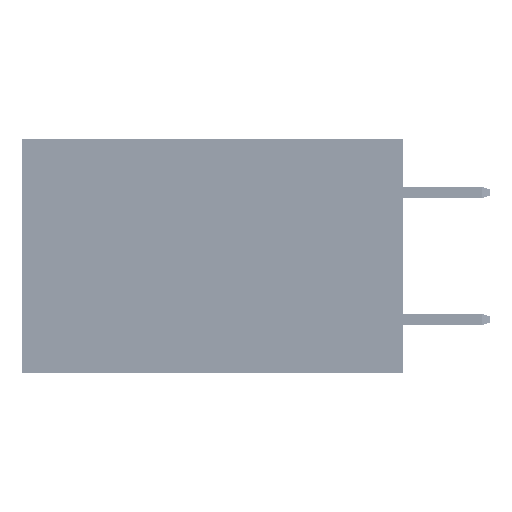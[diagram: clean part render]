
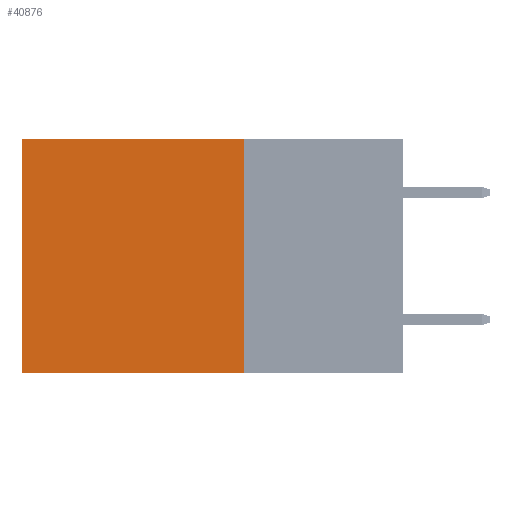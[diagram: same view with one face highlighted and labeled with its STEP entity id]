
A CAD part, left-side view. The second image highlights one B-rep face of the part: STEP entity #40876.
In plain terms, the highlighted planar face has unit normal (-1, 0, 0).
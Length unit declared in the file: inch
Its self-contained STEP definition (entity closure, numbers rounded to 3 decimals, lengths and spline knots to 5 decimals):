
#235 = VERTEX_POINT ( 'NONE', #27423 ) ;
#809 = EDGE_CURVE ( 'NONE', #15833, #235, #5172, .T. ) ;
#906 = CARTESIAN_POINT ( 'NONE',  ( 0.2875, 0.25, 0. ) ) ;
#944 = CARTESIAN_POINT ( 'NONE',  ( 0.2875, 0.25, 0. ) ) ;
#1489 = DIRECTION ( 'NONE',  ( 0., 0., -1. ) ) ;
#1515 = CARTESIAN_POINT ( 'NONE',  ( 0.2875, 0.25, -0.37 ) ) ;
#2453 = ORIENTED_EDGE ( 'NONE', *, *, #28197, .F. ) ;
#3823 = VERTEX_POINT ( 'NONE', #26135 ) ;
#4709 = LINE ( 'NONE', #1515, #15919 ) ;
#4826 = EDGE_LOOP ( 'NONE', ( #23606, #8934, #2453, #17939 ) ) ;
#5172 = LINE ( 'NONE', #35268, #29709 ) ;
#5693 = CARTESIAN_POINT ( 'NONE',  ( 0.2875, 0.25, 0. ) ) ;
#7968 = DIRECTION ( 'NONE',  ( 0., 0., -1. ) ) ;
#8451 = CARTESIAN_POINT ( 'NONE',  ( 0.2875, 0.25, 0. ) ) ;
#8521 = LINE ( 'NONE', #906, #23841 ) ;
#8934 = ORIENTED_EDGE ( 'NONE', *, *, #21193, .F. ) ;
#12122 = PLANE ( 'NONE',  #23232 ) ;
#14660 = VECTOR ( 'NONE', #19753, 39.37008 ) ;
#15833 = VERTEX_POINT ( 'NONE', #41503 ) ;
#15919 = VECTOR ( 'NONE', #41958, 39.37008 ) ;
#17939 = ORIENTED_EDGE ( 'NONE', *, *, #20357, .T. ) ;
#18183 = VERTEX_POINT ( 'NONE', #944 ) ;
#19753 = DIRECTION ( 'NONE',  ( 0., 0., -1. ) ) ;
#20357 = EDGE_CURVE ( 'NONE', #18183, #15833, #8521, .T. ) ;
#21193 = EDGE_CURVE ( 'NONE', #3823, #235, #4709, .T. ) ;
#23232 = AXIS2_PLACEMENT_3D ( 'NONE', #8451, #45182, #7968 ) ;
#23606 = ORIENTED_EDGE ( 'NONE', *, *, #809, .T. ) ;
#23841 = VECTOR ( 'NONE', #27503, 39.37008 ) ;
#26135 = CARTESIAN_POINT ( 'NONE',  ( 0.2875, 0.25, -0.37 ) ) ;
#27423 = CARTESIAN_POINT ( 'NONE',  ( 0.2875, 0.6, -0.37 ) ) ;
#27503 = DIRECTION ( 'NONE',  ( 0., 1., 0. ) ) ;
#28197 = EDGE_CURVE ( 'NONE', #18183, #3823, #31568, .T. ) ;
#29709 = VECTOR ( 'NONE', #1489, 39.37008 ) ;
#31568 = LINE ( 'NONE', #5693, #14660 ) ;
#35268 = CARTESIAN_POINT ( 'NONE',  ( 0.2875, 0.6, 0. ) ) ;
#38559 = FACE_OUTER_BOUND ( 'NONE', #4826, .T. ) ;
#40876 = ADVANCED_FACE ( 'NONE', ( #38559 ), #12122, .F. ) ;
#41503 = CARTESIAN_POINT ( 'NONE',  ( 0.2875, 0.6, 0. ) ) ;
#41958 = DIRECTION ( 'NONE',  ( 0., 1., 0. ) ) ;
#45182 = DIRECTION ( 'NONE',  ( 1., 0., 0. ) ) ;
